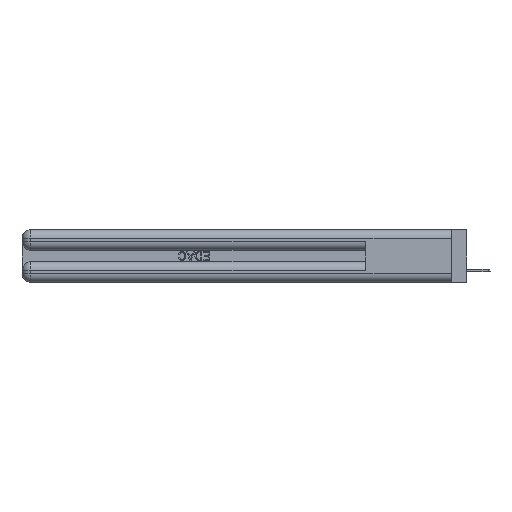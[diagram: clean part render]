
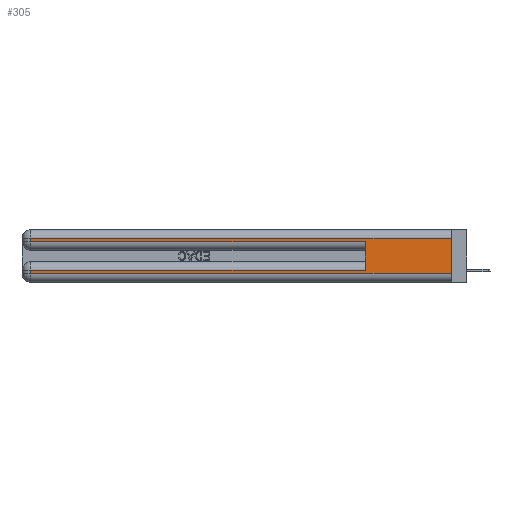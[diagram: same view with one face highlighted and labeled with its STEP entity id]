
A CAD part, left-side view. The second image highlights one B-rep face of the part: STEP entity #305.
In plain terms, the highlighted planar face has unit normal (-1, 0, 0).
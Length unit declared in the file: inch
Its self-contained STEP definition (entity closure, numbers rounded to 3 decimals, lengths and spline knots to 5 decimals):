
#305 = ADVANCED_FACE ( 'NONE', ( #18183 ), #23117, .F. ) ;
#882 = LINE ( 'NONE', #23423, #5780 ) ;
#2599 = DIRECTION ( 'NONE',  ( 0., 0., -1. ) ) ;
#3570 = CARTESIAN_POINT ( 'NONE',  ( 0., 2.94, 0.085 ) ) ;
#3837 = DIRECTION ( 'NONE',  ( 0., 1., 0. ) ) ;
#4035 = EDGE_CURVE ( 'NONE', #26309, #25410, #42042, .T. ) ;
#5258 = DIRECTION ( 'NONE',  ( 0., 1., 0. ) ) ;
#5265 = CARTESIAN_POINT ( 'NONE',  ( 0., 2.94, 0.285 ) ) ;
#5545 = VERTEX_POINT ( 'NONE', #20235 ) ;
#5780 = VECTOR ( 'NONE', #2599, 39.37008 ) ;
#6824 = VERTEX_POINT ( 'NONE', #39680 ) ;
#6996 = LINE ( 'NONE', #15088, #33234 ) ;
#7639 = ORIENTED_EDGE ( 'NONE', *, *, #21377, .T. ) ;
#8489 = CARTESIAN_POINT ( 'NONE',  ( 0., 2.94, 0.37 ) ) ;
#9001 = ORIENTED_EDGE ( 'NONE', *, *, #11428, .T. ) ;
#9243 = CARTESIAN_POINT ( 'NONE',  ( 0., 0., 0.06 ) ) ;
#9302 = LINE ( 'NONE', #9243, #21583 ) ;
#9875 = LINE ( 'NONE', #26016, #28058 ) ;
#9974 = EDGE_LOOP ( 'NONE', ( #18025, #22627, #7639, #9001, #19550, #40574, #21098, #38180 ) ) ;
#11428 = EDGE_CURVE ( 'NONE', #12600, #39426, #13433, .T. ) ;
#11943 = DIRECTION ( 'NONE',  ( 0., -1., 0. ) ) ;
#12503 = CARTESIAN_POINT ( 'NONE',  ( 0., 0., 0.37 ) ) ;
#12600 = VERTEX_POINT ( 'NONE', #5265 ) ;
#13174 = VECTOR ( 'NONE', #17989, 39.37008 ) ;
#13433 = LINE ( 'NONE', #24812, #17138 ) ;
#15088 = CARTESIAN_POINT ( 'NONE',  ( 0., 0., 0.31 ) ) ;
#15695 = EDGE_CURVE ( 'NONE', #36879, #39426, #9875, .T. ) ;
#15712 = EDGE_CURVE ( 'NONE', #25410, #30426, #9302, .T. ) ;
#16445 = LINE ( 'NONE', #8489, #16977 ) ;
#16977 = VECTOR ( 'NONE', #20005, 39.37008 ) ;
#17138 = VECTOR ( 'NONE', #11943, 39.37008 ) ;
#17989 = DIRECTION ( 'NONE',  ( 0., 0., -1. ) ) ;
#18025 = ORIENTED_EDGE ( 'NONE', *, *, #21190, .F. ) ;
#18183 = FACE_OUTER_BOUND ( 'NONE', #9974, .T. ) ;
#19550 = ORIENTED_EDGE ( 'NONE', *, *, #15695, .F. ) ;
#20005 = DIRECTION ( 'NONE',  ( 0., 0., -1. ) ) ;
#20235 = CARTESIAN_POINT ( 'NONE',  ( 0., 2.94, 0.31 ) ) ;
#21098 = ORIENTED_EDGE ( 'NONE', *, *, #4035, .T. ) ;
#21190 = EDGE_CURVE ( 'NONE', #6824, #30426, #882, .T. ) ;
#21377 = EDGE_CURVE ( 'NONE', #5545, #12600, #16445, .T. ) ;
#21516 = EDGE_CURVE ( 'NONE', #36879, #26309, #39477, .T. ) ;
#21583 = VECTOR ( 'NONE', #33962, 39.37008 ) ;
#22415 = CARTESIAN_POINT ( 'NONE',  ( 0., 0., 0.06 ) ) ;
#22627 = ORIENTED_EDGE ( 'NONE', *, *, #27237, .T. ) ;
#22657 = DIRECTION ( 'NONE',  ( 0., 0., -1. ) ) ;
#23117 = PLANE ( 'NONE',  #35715 ) ;
#23423 = CARTESIAN_POINT ( 'NONE',  ( 0., 0., 0.37 ) ) ;
#24812 = CARTESIAN_POINT ( 'NONE',  ( 0., 0., 0.285 ) ) ;
#25410 = VERTEX_POINT ( 'NONE', #39108 ) ;
#26016 = CARTESIAN_POINT ( 'NONE',  ( 0., 0.6, 0.145 ) ) ;
#26309 = VERTEX_POINT ( 'NONE', #3570 ) ;
#27237 = EDGE_CURVE ( 'NONE', #6824, #5545, #6996, .T. ) ;
#28058 = VECTOR ( 'NONE', #39651, 39.37008 ) ;
#30426 = VERTEX_POINT ( 'NONE', #22415 ) ;
#33041 = VECTOR ( 'NONE', #3837, 39.37008 ) ;
#33234 = VECTOR ( 'NONE', #5258, 39.37008 ) ;
#33962 = DIRECTION ( 'NONE',  ( 0., -1., 0. ) ) ;
#34520 = CARTESIAN_POINT ( 'NONE',  ( 0., 2.94, 0.37 ) ) ;
#35715 = AXIS2_PLACEMENT_3D ( 'NONE', #12503, #40072, #22657 ) ;
#35733 = CARTESIAN_POINT ( 'NONE',  ( 0., 0.6, 0.285 ) ) ;
#35863 = CARTESIAN_POINT ( 'NONE',  ( 0., 0.6, 0.085 ) ) ;
#36879 = VERTEX_POINT ( 'NONE', #35863 ) ;
#37951 = CARTESIAN_POINT ( 'NONE',  ( 0., 0., 0.085 ) ) ;
#38180 = ORIENTED_EDGE ( 'NONE', *, *, #15712, .T. ) ;
#39108 = CARTESIAN_POINT ( 'NONE',  ( 0., 2.94, 0.06 ) ) ;
#39426 = VERTEX_POINT ( 'NONE', #35733 ) ;
#39477 = LINE ( 'NONE', #37951, #33041 ) ;
#39651 = DIRECTION ( 'NONE',  ( 0., 0., 1. ) ) ;
#39680 = CARTESIAN_POINT ( 'NONE',  ( 0., 0., 0.31 ) ) ;
#40072 = DIRECTION ( 'NONE',  ( 1., 0., 0. ) ) ;
#40574 = ORIENTED_EDGE ( 'NONE', *, *, #21516, .T. ) ;
#42042 = LINE ( 'NONE', #34520, #13174 ) ;
